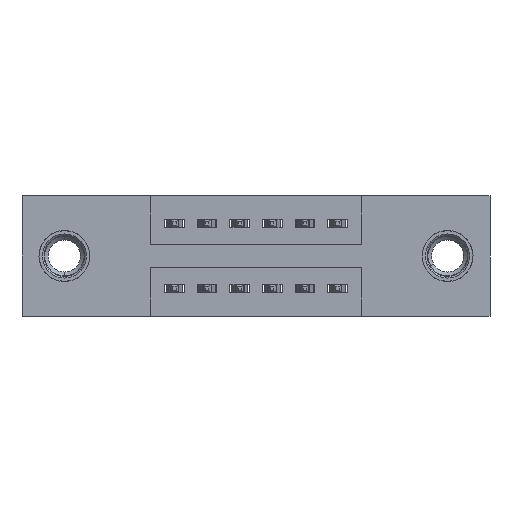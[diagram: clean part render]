
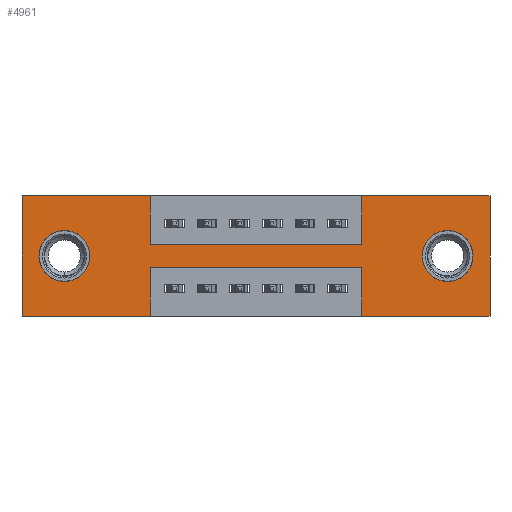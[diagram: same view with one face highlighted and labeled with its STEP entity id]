
A CAD part, front view. The second image highlights one B-rep face of the part: STEP entity #4961.
In plain terms, the highlighted planar face has unit normal (0, -1, 0).
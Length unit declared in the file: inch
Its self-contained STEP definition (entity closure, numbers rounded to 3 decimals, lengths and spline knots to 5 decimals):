
#48 = EDGE_CURVE ( 'NONE', #6059, #9143, #453, .T. ) ;
#104 = AXIS2_PLACEMENT_3D ( 'NONE', #5930, #1831, #1030 ) ;
#108 = VERTEX_POINT ( 'NONE', #2546 ) ;
#116 = DIRECTION ( 'NONE',  ( 0., 1., 0. ) ) ;
#254 = CARTESIAN_POINT ( 'NONE',  ( 0., 0., -0.37 ) ) ;
#330 = CARTESIAN_POINT ( 'NONE',  ( 0.13, 0., -0.185 ) ) ;
#453 = CIRCLE ( 'NONE', #4723, 0.078 ) ;
#741 = ORIENTED_EDGE ( 'NONE', *, *, #5109, .F. ) ;
#796 = LINE ( 'NONE', #4073, #1582 ) ;
#1030 = DIRECTION ( 'NONE',  ( 0., 0., -1. ) ) ;
#1038 = CARTESIAN_POINT ( 'NONE',  ( 1.435, 0., 0. ) ) ;
#1138 = LINE ( 'NONE', #5409, #6205 ) ;
#1351 = LINE ( 'NONE', #3841, #4992 ) ;
#1471 = ORIENTED_EDGE ( 'NONE', *, *, #4984, .F. ) ;
#1490 = CARTESIAN_POINT ( 'NONE',  ( 1.305, 0., -0.185 ) ) ;
#1518 = ORIENTED_EDGE ( 'NONE', *, *, #2255, .T. ) ;
#1582 = VECTOR ( 'NONE', #4914, 39.37008 ) ;
#1831 = DIRECTION ( 'NONE',  ( 0., -1., 0. ) ) ;
#1897 = DIRECTION ( 'NONE',  ( -1., 0., 0. ) ) ;
#1911 = EDGE_CURVE ( 'NONE', #9143, #6059, #2109, .T. ) ;
#1992 = EDGE_LOOP ( 'NONE', ( #1518, #7632 ) ) ;
#2074 = DIRECTION ( 'NONE',  ( 1., 0., 0. ) ) ;
#2095 = DIRECTION ( 'NONE',  ( 0., 0., 1. ) ) ;
#2109 = CIRCLE ( 'NONE', #6543, 0.078 ) ;
#2203 = EDGE_CURVE ( 'NONE', #10630, #4340, #2247, .T. ) ;
#2216 = VERTEX_POINT ( 'NONE', #6393 ) ;
#2247 = LINE ( 'NONE', #5244, #3401 ) ;
#2255 = EDGE_CURVE ( 'NONE', #4249, #7839, #3936, .T. ) ;
#2276 = DIRECTION ( 'NONE',  ( 0., 0., -1. ) ) ;
#2546 = CARTESIAN_POINT ( 'NONE',  ( 1.0425, 0., -0.15 ) ) ;
#2601 = DIRECTION ( 'NONE',  ( 0., 0., -1. ) ) ;
#2610 = ORIENTED_EDGE ( 'NONE', *, *, #8175, .F. ) ;
#2876 = VERTEX_POINT ( 'NONE', #8506 ) ;
#2947 = EDGE_CURVE ( 'NONE', #3849, #6601, #796, .T. ) ;
#2958 = FACE_BOUND ( 'NONE', #1992, .T. ) ;
#3000 = LINE ( 'NONE', #3341, #10013 ) ;
#3051 = EDGE_CURVE ( 'NONE', #2216, #8152, #3000, .T. ) ;
#3173 = CARTESIAN_POINT ( 'NONE',  ( 0., 0., 0. ) ) ;
#3341 = CARTESIAN_POINT ( 'NONE',  ( 0., 0., -0.37 ) ) ;
#3401 = VECTOR ( 'NONE', #2095, 39.37008 ) ;
#3529 = DIRECTION ( 'NONE',  ( 0., 0., -1. ) ) ;
#3543 = EDGE_LOOP ( 'NONE', ( #8207, #5903 ) ) ;
#3562 = DIRECTION ( 'NONE',  ( 0., 1., 0. ) ) ;
#3719 = ORIENTED_EDGE ( 'NONE', *, *, #3051, .F. ) ;
#3726 = FACE_OUTER_BOUND ( 'NONE', #8671, .T. ) ;
#3781 = EDGE_CURVE ( 'NONE', #8152, #6258, #4668, .T. ) ;
#3812 = CARTESIAN_POINT ( 'NONE',  ( 1.0425, 0., -0.37 ) ) ;
#3820 = CARTESIAN_POINT ( 'NONE',  ( 0.3925, 0., -0.15 ) ) ;
#3841 = CARTESIAN_POINT ( 'NONE',  ( 1.0425, 0., 0. ) ) ;
#3849 = VERTEX_POINT ( 'NONE', #7000 ) ;
#3936 = CIRCLE ( 'NONE', #8257, 0.078 ) ;
#4073 = CARTESIAN_POINT ( 'NONE',  ( 0., 0., 0. ) ) ;
#4111 = CARTESIAN_POINT ( 'NONE',  ( 1.0425, 0., -0.37 ) ) ;
#4227 = EDGE_CURVE ( 'NONE', #4340, #2876, #1138, .T. ) ;
#4249 = VERTEX_POINT ( 'NONE', #10312 ) ;
#4340 = VERTEX_POINT ( 'NONE', #3173 ) ;
#4350 = CARTESIAN_POINT ( 'NONE',  ( 1.435, 0., 0. ) ) ;
#4378 = VECTOR ( 'NONE', #1897, 39.37008 ) ;
#4404 = DIRECTION ( 'NONE',  ( 0., 0., 1. ) ) ;
#4668 = LINE ( 'NONE', #3812, #8863 ) ;
#4723 = AXIS2_PLACEMENT_3D ( 'NONE', #330, #3562, #4404 ) ;
#4776 = ORIENTED_EDGE ( 'NONE', *, *, #4227, .F. ) ;
#4845 = CARTESIAN_POINT ( 'NONE',  ( 0.13, 0., -0.263 ) ) ;
#4914 = DIRECTION ( 'NONE',  ( 1., 0., 0. ) ) ;
#4961 = ADVANCED_FACE ( 'NONE', ( #2958, #6597, #3726 ), #5040, .T. ) ;
#4984 = EDGE_CURVE ( 'NONE', #6258, #10719, #7672, .T. ) ;
#4992 = VECTOR ( 'NONE', #10463, 39.37008 ) ;
#5040 = PLANE ( 'NONE',  #104 ) ;
#5072 = DIRECTION ( 'NONE',  ( -1., 0., 0. ) ) ;
#5078 = VECTOR ( 'NONE', #7410, 39.37008 ) ;
#5109 = EDGE_CURVE ( 'NONE', #2876, #5477, #10227, .T. ) ;
#5163 = CARTESIAN_POINT ( 'NONE',  ( 0.13, 0., -0.107 ) ) ;
#5244 = CARTESIAN_POINT ( 'NONE',  ( 0., 0., 0. ) ) ;
#5409 = CARTESIAN_POINT ( 'NONE',  ( 0., 0., 0. ) ) ;
#5477 = VERTEX_POINT ( 'NONE', #6063 ) ;
#5545 = VECTOR ( 'NONE', #9334, 39.37008 ) ;
#5866 = EDGE_CURVE ( 'NONE', #10719, #6935, #7779, .T. ) ;
#5903 = ORIENTED_EDGE ( 'NONE', *, *, #1911, .T. ) ;
#5930 = CARTESIAN_POINT ( 'NONE',  ( 0., 0., -0.37 ) ) ;
#6031 = DIRECTION ( 'NONE',  ( 0., 0., -1. ) ) ;
#6059 = VERTEX_POINT ( 'NONE', #5163 ) ;
#6063 = CARTESIAN_POINT ( 'NONE',  ( 0.3925, 0., -0.15 ) ) ;
#6205 = VECTOR ( 'NONE', #9639, 39.37008 ) ;
#6258 = VERTEX_POINT ( 'NONE', #7882 ) ;
#6302 = CARTESIAN_POINT ( 'NONE',  ( 0.3925, 0., 0. ) ) ;
#6393 = CARTESIAN_POINT ( 'NONE',  ( 1.435, 0., -0.37 ) ) ;
#6476 = CARTESIAN_POINT ( 'NONE',  ( 1.305, 0., -0.263 ) ) ;
#6543 = AXIS2_PLACEMENT_3D ( 'NONE', #10432, #7960, #9523 ) ;
#6576 = VECTOR ( 'NONE', #2601, 39.37008 ) ;
#6597 = FACE_BOUND ( 'NONE', #3543, .T. ) ;
#6601 = VERTEX_POINT ( 'NONE', #1038 ) ;
#6639 = EDGE_CURVE ( 'NONE', #6601, #2216, #9430, .T. ) ;
#6935 = VERTEX_POINT ( 'NONE', #9622 ) ;
#7000 = CARTESIAN_POINT ( 'NONE',  ( 1.0425, 0., 0. ) ) ;
#7078 = CIRCLE ( 'NONE', #8437, 0.078 ) ;
#7119 = ORIENTED_EDGE ( 'NONE', *, *, #2203, .F. ) ;
#7410 = DIRECTION ( 'NONE',  ( -1., 0., 0. ) ) ;
#7418 = VECTOR ( 'NONE', #2276, 39.37008 ) ;
#7632 = ORIENTED_EDGE ( 'NONE', *, *, #7660, .T. ) ;
#7660 = EDGE_CURVE ( 'NONE', #7839, #4249, #7078, .T. ) ;
#7672 = LINE ( 'NONE', #10186, #4378 ) ;
#7761 = ORIENTED_EDGE ( 'NONE', *, *, #3781, .F. ) ;
#7779 = LINE ( 'NONE', #9023, #5545 ) ;
#7832 = ORIENTED_EDGE ( 'NONE', *, *, #9419, .F. ) ;
#7839 = VERTEX_POINT ( 'NONE', #6476 ) ;
#7882 = CARTESIAN_POINT ( 'NONE',  ( 1.0425, 0., -0.22 ) ) ;
#7960 = DIRECTION ( 'NONE',  ( 0., 1., 0. ) ) ;
#7982 = LINE ( 'NONE', #3820, #8601 ) ;
#8123 = ORIENTED_EDGE ( 'NONE', *, *, #9133, .F. ) ;
#8152 = VERTEX_POINT ( 'NONE', #4111 ) ;
#8175 = EDGE_CURVE ( 'NONE', #108, #3849, #1351, .T. ) ;
#8207 = ORIENTED_EDGE ( 'NONE', *, *, #48, .T. ) ;
#8252 = ORIENTED_EDGE ( 'NONE', *, *, #2947, .F. ) ;
#8257 = AXIS2_PLACEMENT_3D ( 'NONE', #1490, #116, #6031 ) ;
#8437 = AXIS2_PLACEMENT_3D ( 'NONE', #10222, #10324, #3529 ) ;
#8497 = ORIENTED_EDGE ( 'NONE', *, *, #5866, .F. ) ;
#8506 = CARTESIAN_POINT ( 'NONE',  ( 0.3925, 0., 0. ) ) ;
#8601 = VECTOR ( 'NONE', #2074, 39.37008 ) ;
#8671 = EDGE_LOOP ( 'NONE', ( #8497, #1471, #7761, #3719, #9424, #8252, #2610, #7832, #741, #4776, #7119, #8123 ) ) ;
#8753 = LINE ( 'NONE', #10721, #5078 ) ;
#8863 = VECTOR ( 'NONE', #10584, 39.37008 ) ;
#9023 = CARTESIAN_POINT ( 'NONE',  ( 0.3925, 0., -0.37 ) ) ;
#9133 = EDGE_CURVE ( 'NONE', #6935, #10630, #8753, .T. ) ;
#9143 = VERTEX_POINT ( 'NONE', #4845 ) ;
#9334 = DIRECTION ( 'NONE',  ( 0., 0., -1. ) ) ;
#9419 = EDGE_CURVE ( 'NONE', #5477, #108, #7982, .T. ) ;
#9424 = ORIENTED_EDGE ( 'NONE', *, *, #6639, .F. ) ;
#9430 = LINE ( 'NONE', #4350, #6576 ) ;
#9523 = DIRECTION ( 'NONE',  ( 0., 0., 1. ) ) ;
#9622 = CARTESIAN_POINT ( 'NONE',  ( 0.3925, 0., -0.37 ) ) ;
#9639 = DIRECTION ( 'NONE',  ( 1., 0., 0. ) ) ;
#10013 = VECTOR ( 'NONE', #5072, 39.37008 ) ;
#10186 = CARTESIAN_POINT ( 'NONE',  ( 0.3925, 0., -0.22 ) ) ;
#10222 = CARTESIAN_POINT ( 'NONE',  ( 1.305, 0., -0.185 ) ) ;
#10227 = LINE ( 'NONE', #6302, #7418 ) ;
#10312 = CARTESIAN_POINT ( 'NONE',  ( 1.305, 0., -0.107 ) ) ;
#10324 = DIRECTION ( 'NONE',  ( 0., 1., 0. ) ) ;
#10432 = CARTESIAN_POINT ( 'NONE',  ( 0.13, 0., -0.185 ) ) ;
#10463 = DIRECTION ( 'NONE',  ( 0., 0., 1. ) ) ;
#10584 = DIRECTION ( 'NONE',  ( 0., 0., 1. ) ) ;
#10630 = VERTEX_POINT ( 'NONE', #254 ) ;
#10673 = CARTESIAN_POINT ( 'NONE',  ( 0.3925, 0., -0.22 ) ) ;
#10719 = VERTEX_POINT ( 'NONE', #10673 ) ;
#10721 = CARTESIAN_POINT ( 'NONE',  ( 0., 0., -0.37 ) ) ;
